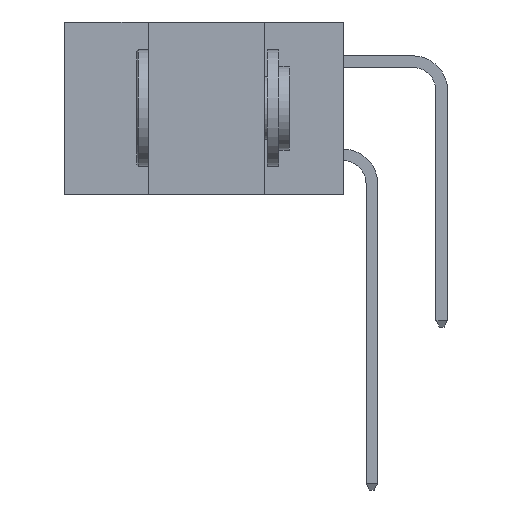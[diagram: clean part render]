
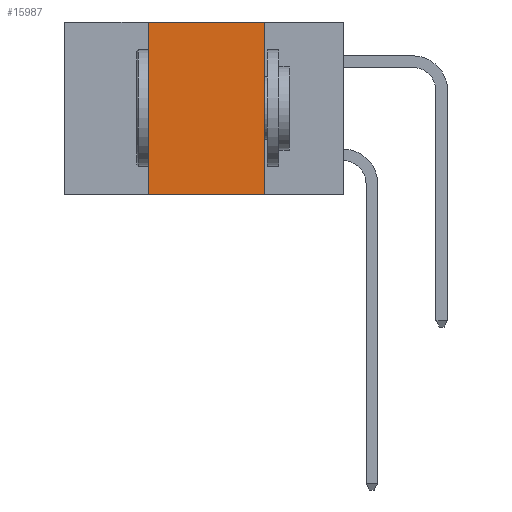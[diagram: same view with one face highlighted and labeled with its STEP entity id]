
A CAD part, left-side view. The second image highlights one B-rep face of the part: STEP entity #15987.
In plain terms, the highlighted planar face has unit normal (-1, 0, 0).
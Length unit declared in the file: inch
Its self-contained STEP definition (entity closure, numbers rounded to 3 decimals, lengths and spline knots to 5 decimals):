
#172 = FACE_OUTER_BOUND ( 'NONE', #25720, .T. ) ;
#288 = CARTESIAN_POINT ( 'NONE',  ( 0., 0.42, -0.37 ) ) ;
#972 = LINE ( 'NONE', #27387, #23462 ) ;
#1409 = DIRECTION ( 'NONE',  ( 0., -1., 0. ) ) ;
#3178 = CARTESIAN_POINT ( 'NONE',  ( 0., 0.6, -0.37 ) ) ;
#3530 = LINE ( 'NONE', #288, #14551 ) ;
#3652 = PLANE ( 'NONE',  #9396 ) ;
#5553 = CARTESIAN_POINT ( 'NONE',  ( 0., 0.42, 0. ) ) ;
#5921 = DIRECTION ( 'NONE',  ( 1., 0., 0. ) ) ;
#6019 = ORIENTED_EDGE ( 'NONE', *, *, #19096, .F. ) ;
#8881 = EDGE_CURVE ( 'NONE', #22428, #18893, #20943, .T. ) ;
#9396 = AXIS2_PLACEMENT_3D ( 'NONE', #18978, #5921, #21128 ) ;
#9410 = VECTOR ( 'NONE', #12003, 39.37008 ) ;
#10095 = CARTESIAN_POINT ( 'NONE',  ( 0., 0.42, -0.37 ) ) ;
#10894 = CARTESIAN_POINT ( 'NONE',  ( 0., 0.17, -0.37 ) ) ;
#12003 = DIRECTION ( 'NONE',  ( 0., -1., 0. ) ) ;
#14191 = LINE ( 'NONE', #10894, #18571 ) ;
#14551 = VECTOR ( 'NONE', #22137, 39.37008 ) ;
#14668 = CARTESIAN_POINT ( 'NONE',  ( 0., 0.17, -0.37 ) ) ;
#14972 = ORIENTED_EDGE ( 'NONE', *, *, #8881, .T. ) ;
#15987 = ADVANCED_FACE ( 'NONE', ( #172 ), #3652, .F. ) ;
#17138 = VERTEX_POINT ( 'NONE', #5553 ) ;
#17590 = EDGE_CURVE ( 'NONE', #22428, #17138, #3530, .T. ) ;
#17794 = CARTESIAN_POINT ( 'NONE',  ( 0., 0.17, 0. ) ) ;
#18571 = VECTOR ( 'NONE', #19478, 39.37008 ) ;
#18893 = VERTEX_POINT ( 'NONE', #14668 ) ;
#18978 = CARTESIAN_POINT ( 'NONE',  ( 0., 0.6, 0. ) ) ;
#19096 = EDGE_CURVE ( 'NONE', #23994, #18893, #14191, .T. ) ;
#19478 = DIRECTION ( 'NONE',  ( 0., 0., -1. ) ) ;
#19660 = ORIENTED_EDGE ( 'NONE', *, *, #17590, .F. ) ;
#19988 = ORIENTED_EDGE ( 'NONE', *, *, #24750, .F. ) ;
#20943 = LINE ( 'NONE', #3178, #9410 ) ;
#21128 = DIRECTION ( 'NONE',  ( 0., 0., -1. ) ) ;
#22137 = DIRECTION ( 'NONE',  ( 0., 0., 1. ) ) ;
#22428 = VERTEX_POINT ( 'NONE', #10095 ) ;
#23462 = VECTOR ( 'NONE', #1409, 39.37008 ) ;
#23994 = VERTEX_POINT ( 'NONE', #17794 ) ;
#24750 = EDGE_CURVE ( 'NONE', #17138, #23994, #972, .T. ) ;
#25720 = EDGE_LOOP ( 'NONE', ( #6019, #19988, #19660, #14972 ) ) ;
#27387 = CARTESIAN_POINT ( 'NONE',  ( 0., 0.6, 0. ) ) ;
